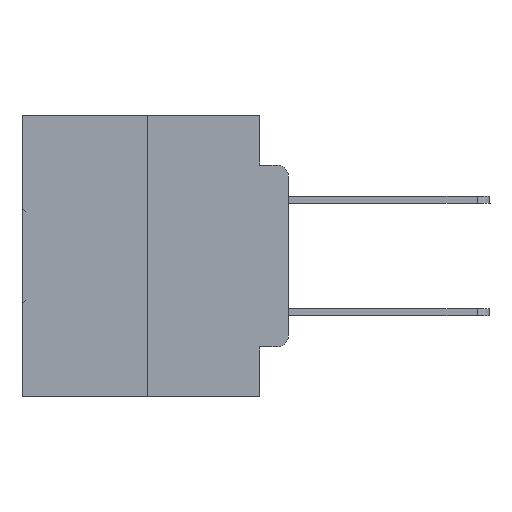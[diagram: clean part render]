
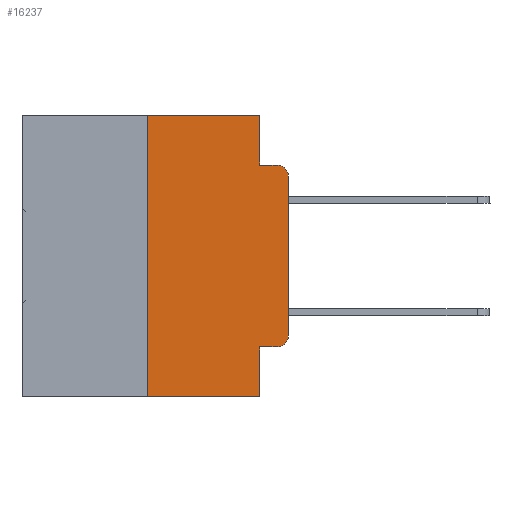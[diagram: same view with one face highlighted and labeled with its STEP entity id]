
A CAD part, left-side view. The second image highlights one B-rep face of the part: STEP entity #16237.
In plain terms, the highlighted planar face has unit normal (-1, 0, 0).
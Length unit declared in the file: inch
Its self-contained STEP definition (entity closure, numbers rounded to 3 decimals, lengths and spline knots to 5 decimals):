
#634 = VECTOR ( 'NONE', #15046, 39.37008 ) ;
#889 = CARTESIAN_POINT ( 'NONE',  ( 0., 0.25, 0. ) ) ;
#1505 = VECTOR ( 'NONE', #15107, 39.37008 ) ;
#1559 = DIRECTION ( 'NONE',  ( 0., 0., -1. ) ) ;
#1574 = LINE ( 'NONE', #889, #6723 ) ;
#1623 = DIRECTION ( 'NONE',  ( 0., 0., -1. ) ) ;
#1642 = FACE_OUTER_BOUND ( 'NONE', #12628, .T. ) ;
#1875 = EDGE_CURVE ( 'NONE', #22259, #23481, #24739, .T. ) ;
#1970 = CARTESIAN_POINT ( 'NONE',  ( 0., 0., -0.3915 ) ) ;
#2946 = LINE ( 'NONE', #14205, #29015 ) ;
#3357 = CARTESIAN_POINT ( 'NONE',  ( 0., 0.02, -0.1085 ) ) ;
#3902 = VECTOR ( 'NONE', #31495, 39.37008 ) ;
#4217 = CARTESIAN_POINT ( 'NONE',  ( 0., 0.473, -0.5 ) ) ;
#4746 = DIRECTION ( 'NONE',  ( 0., -1., 0. ) ) ;
#5198 = VECTOR ( 'NONE', #31379, 39.37008 ) ;
#5835 = CARTESIAN_POINT ( 'NONE',  ( 0., 0.051, 0. ) ) ;
#5890 = DIRECTION ( 'NONE',  ( 0., 0., -1. ) ) ;
#6554 = AXIS2_PLACEMENT_3D ( 'NONE', #31783, #16812, #1559 ) ;
#6723 = VECTOR ( 'NONE', #8552, 39.37008 ) ;
#7167 = ORIENTED_EDGE ( 'NONE', *, *, #27875, .F. ) ;
#7168 = EDGE_CURVE ( 'NONE', #12383, #15000, #2946, .T. ) ;
#7412 = CARTESIAN_POINT ( 'NONE',  ( 0., 0.051, 0. ) ) ;
#8067 = AXIS2_PLACEMENT_3D ( 'NONE', #3357, #21075, #5890 ) ;
#8552 = DIRECTION ( 'NONE',  ( 0., 0., 1. ) ) ;
#8620 = VERTEX_POINT ( 'NONE', #1970 ) ;
#8760 = VERTEX_POINT ( 'NONE', #32698 ) ;
#9151 = DIRECTION ( 'NONE',  ( 0., -1., 0. ) ) ;
#9171 = PLANE ( 'NONE',  #25741 ) ;
#9555 = ORIENTED_EDGE ( 'NONE', *, *, #19459, .F. ) ;
#9947 = ORIENTED_EDGE ( 'NONE', *, *, #21551, .T. ) ;
#10024 = VERTEX_POINT ( 'NONE', #14522 ) ;
#10620 = EDGE_CURVE ( 'NONE', #15000, #8620, #30390, .T. ) ;
#11396 = EDGE_CURVE ( 'NONE', #11606, #10024, #21738, .T. ) ;
#11606 = VERTEX_POINT ( 'NONE', #5835 ) ;
#11721 = EDGE_CURVE ( 'NONE', #32025, #11606, #17417, .T. ) ;
#12383 = VERTEX_POINT ( 'NONE', #24074 ) ;
#12628 = EDGE_LOOP ( 'NONE', ( #27710, #9947, #30041, #24966, #19863, #7167, #27327, #9555, #29670, #30444 ) ) ;
#14205 = CARTESIAN_POINT ( 'NONE',  ( 0., 0.051, -0.4115 ) ) ;
#14522 = CARTESIAN_POINT ( 'NONE',  ( 0., 0.051, -0.0885 ) ) ;
#15000 = VERTEX_POINT ( 'NONE', #20626 ) ;
#15046 = DIRECTION ( 'NONE',  ( 0., 0., -1. ) ) ;
#15107 = DIRECTION ( 'NONE',  ( 0., 0., -1. ) ) ;
#15154 = CARTESIAN_POINT ( 'NONE',  ( 0., 0.051, 0. ) ) ;
#15201 = CARTESIAN_POINT ( 'NONE',  ( 0., 0.25, -0.5 ) ) ;
#15439 = VECTOR ( 'NONE', #4746, 39.37008 ) ;
#16237 = ADVANCED_FACE ( 'NONE', ( #1642 ), #9171, .F. ) ;
#16748 = EDGE_CURVE ( 'NONE', #8620, #28997, #20257, .T. ) ;
#16812 = DIRECTION ( 'NONE',  ( -1., 0., 0. ) ) ;
#16876 = DIRECTION ( 'NONE',  ( 1., 0., 0. ) ) ;
#17417 = LINE ( 'NONE', #21463, #3902 ) ;
#18059 = CARTESIAN_POINT ( 'NONE',  ( 0., 0., -0.1085 ) ) ;
#18177 = EDGE_CURVE ( 'NONE', #10024, #8760, #28015, .T. ) ;
#18850 = VECTOR ( 'NONE', #19280, 39.37008 ) ;
#19280 = DIRECTION ( 'NONE',  ( 0., -1., 0. ) ) ;
#19459 = EDGE_CURVE ( 'NONE', #12383, #23481, #21694, .T. ) ;
#19863 = ORIENTED_EDGE ( 'NONE', *, *, #11721, .F. ) ;
#19918 = CARTESIAN_POINT ( 'NONE',  ( 0., 0.051, -0.0885 ) ) ;
#20257 = LINE ( 'NONE', #28989, #5198 ) ;
#20626 = CARTESIAN_POINT ( 'NONE',  ( 0., 0.02, -0.4115 ) ) ;
#21075 = DIRECTION ( 'NONE',  ( -1., 0., 0. ) ) ;
#21463 = CARTESIAN_POINT ( 'NONE',  ( 0., 0.473, 0. ) ) ;
#21551 = EDGE_CURVE ( 'NONE', #28997, #8760, #24670, .T. ) ;
#21694 = LINE ( 'NONE', #15154, #634 ) ;
#21738 = LINE ( 'NONE', #7412, #1505 ) ;
#22259 = VERTEX_POINT ( 'NONE', #15201 ) ;
#23481 = VERTEX_POINT ( 'NONE', #27756 ) ;
#24074 = CARTESIAN_POINT ( 'NONE',  ( 0., 0.051, -0.4115 ) ) ;
#24670 = CIRCLE ( 'NONE', #8067, 0.02 ) ;
#24739 = LINE ( 'NONE', #4217, #18850 ) ;
#24966 = ORIENTED_EDGE ( 'NONE', *, *, #11396, .F. ) ;
#25741 = AXIS2_PLACEMENT_3D ( 'NONE', #26847, #16876, #1623 ) ;
#26847 = CARTESIAN_POINT ( 'NONE',  ( 0., 0.473, 0. ) ) ;
#27151 = CARTESIAN_POINT ( 'NONE',  ( 0., 0.25, 0. ) ) ;
#27327 = ORIENTED_EDGE ( 'NONE', *, *, #1875, .T. ) ;
#27710 = ORIENTED_EDGE ( 'NONE', *, *, #16748, .T. ) ;
#27756 = CARTESIAN_POINT ( 'NONE',  ( 0., 0.051, -0.5 ) ) ;
#27875 = EDGE_CURVE ( 'NONE', #22259, #32025, #1574, .T. ) ;
#28015 = LINE ( 'NONE', #19918, #15439 ) ;
#28989 = CARTESIAN_POINT ( 'NONE',  ( 0., 0., 0. ) ) ;
#28997 = VERTEX_POINT ( 'NONE', #18059 ) ;
#29015 = VECTOR ( 'NONE', #9151, 39.37008 ) ;
#29670 = ORIENTED_EDGE ( 'NONE', *, *, #7168, .T. ) ;
#30041 = ORIENTED_EDGE ( 'NONE', *, *, #18177, .F. ) ;
#30390 = CIRCLE ( 'NONE', #6554, 0.02 ) ;
#30444 = ORIENTED_EDGE ( 'NONE', *, *, #10620, .T. ) ;
#31379 = DIRECTION ( 'NONE',  ( 0., 0., 1. ) ) ;
#31495 = DIRECTION ( 'NONE',  ( 0., -1., 0. ) ) ;
#31783 = CARTESIAN_POINT ( 'NONE',  ( 0., 0.02, -0.3915 ) ) ;
#32025 = VERTEX_POINT ( 'NONE', #27151 ) ;
#32698 = CARTESIAN_POINT ( 'NONE',  ( 0., 0.02, -0.0885 ) ) ;
